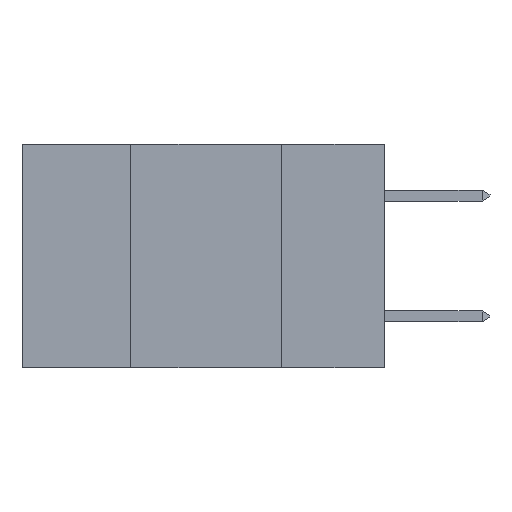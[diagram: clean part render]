
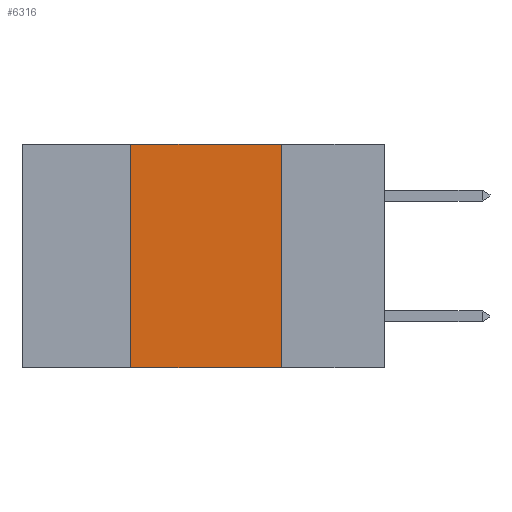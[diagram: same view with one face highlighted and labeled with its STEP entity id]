
A CAD part, left-side view. The second image highlights one B-rep face of the part: STEP entity #6316.
In plain terms, the highlighted planar face has unit normal (-1, 0, 0).
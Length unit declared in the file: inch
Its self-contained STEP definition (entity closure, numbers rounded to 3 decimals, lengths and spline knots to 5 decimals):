
#10 = CARTESIAN_POINT ( 'NONE',  ( 0., 0.17, 0. ) ) ;
#53 = LINE ( 'NONE', #8940, #2990 ) ;
#350 = ORIENTED_EDGE ( 'NONE', *, *, #14441, .F. ) ;
#822 = EDGE_CURVE ( 'NONE', #12774, #11221, #4454, .T. ) ;
#985 = VECTOR ( 'NONE', #1012, 39.37008 ) ;
#1012 = DIRECTION ( 'NONE',  ( 0., -1., 0. ) ) ;
#1307 = DIRECTION ( 'NONE',  ( 0., 0., -1. ) ) ;
#1725 = DIRECTION ( 'NONE',  ( 0., -1., 0. ) ) ;
#1795 = ORIENTED_EDGE ( 'NONE', *, *, #822, .F. ) ;
#1797 = ORIENTED_EDGE ( 'NONE', *, *, #3441, .F. ) ;
#2774 = CARTESIAN_POINT ( 'NONE',  ( 0., 0.42, 0. ) ) ;
#2842 = EDGE_LOOP ( 'NONE', ( #350, #1797, #1795, #8634 ) ) ;
#2990 = VECTOR ( 'NONE', #1725, 39.37008 ) ;
#3441 = EDGE_CURVE ( 'NONE', #11221, #13639, #7574, .T. ) ;
#4230 = CARTESIAN_POINT ( 'NONE',  ( 0., 0.6, 0. ) ) ;
#4454 = LINE ( 'NONE', #2774, #8001 ) ;
#5774 = AXIS2_PLACEMENT_3D ( 'NONE', #4230, #13790, #6662 ) ;
#6013 = CARTESIAN_POINT ( 'NONE',  ( 0., 0.17, 0. ) ) ;
#6082 = VERTEX_POINT ( 'NONE', #10801 ) ;
#6273 = DIRECTION ( 'NONE',  ( 0., 0., 1. ) ) ;
#6316 = ADVANCED_FACE ( 'NONE', ( #14205 ), #12599, .F. ) ;
#6479 = LINE ( 'NONE', #10, #15529 ) ;
#6662 = DIRECTION ( 'NONE',  ( 0., 0., -1. ) ) ;
#7574 = LINE ( 'NONE', #8355, #985 ) ;
#7934 = CARTESIAN_POINT ( 'NONE',  ( 0., 0.42, -0.37 ) ) ;
#8001 = VECTOR ( 'NONE', #6273, 39.37008 ) ;
#8355 = CARTESIAN_POINT ( 'NONE',  ( 0., 0.6, 0. ) ) ;
#8435 = EDGE_CURVE ( 'NONE', #12774, #6082, #53, .T. ) ;
#8634 = ORIENTED_EDGE ( 'NONE', *, *, #8435, .T. ) ;
#8940 = CARTESIAN_POINT ( 'NONE',  ( 0., 0.6, -0.37 ) ) ;
#10801 = CARTESIAN_POINT ( 'NONE',  ( 0., 0.17, -0.37 ) ) ;
#11221 = VERTEX_POINT ( 'NONE', #15119 ) ;
#12599 = PLANE ( 'NONE',  #5774 ) ;
#12774 = VERTEX_POINT ( 'NONE', #7934 ) ;
#13639 = VERTEX_POINT ( 'NONE', #6013 ) ;
#13790 = DIRECTION ( 'NONE',  ( 1., 0., 0. ) ) ;
#14205 = FACE_OUTER_BOUND ( 'NONE', #2842, .T. ) ;
#14441 = EDGE_CURVE ( 'NONE', #13639, #6082, #6479, .T. ) ;
#15119 = CARTESIAN_POINT ( 'NONE',  ( 0., 0.42, 0. ) ) ;
#15529 = VECTOR ( 'NONE', #1307, 39.37008 ) ;
